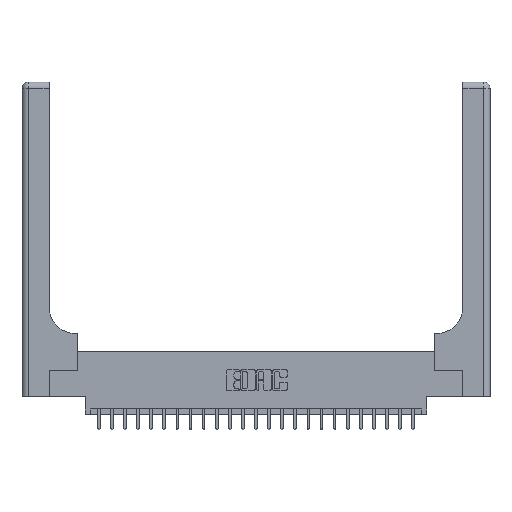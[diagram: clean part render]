
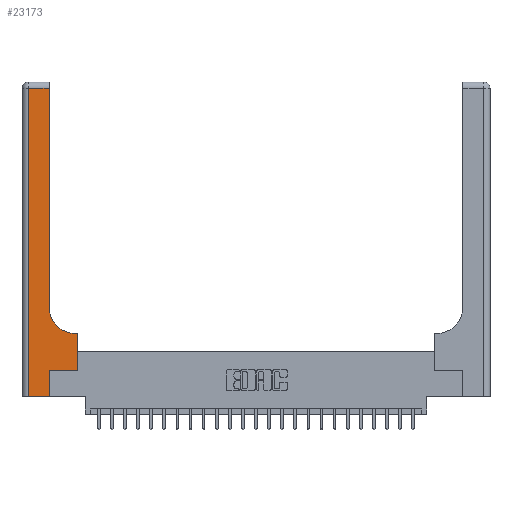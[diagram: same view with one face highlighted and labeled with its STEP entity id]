
A CAD part, top view. The second image highlights one B-rep face of the part: STEP entity #23173.
In plain terms, the highlighted planar face has unit normal (0, 0, 1).
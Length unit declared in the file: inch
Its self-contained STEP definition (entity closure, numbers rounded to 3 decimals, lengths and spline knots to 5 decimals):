
#363 = VECTOR ( 'NONE', #8334, 39.37008 ) ;
#521 = ORIENTED_EDGE ( 'NONE', *, *, #23786, .T. ) ;
#613 = CARTESIAN_POINT ( 'NONE',  ( 0.265, 0., 0.37 ) ) ;
#946 = VERTEX_POINT ( 'NONE', #2927 ) ;
#1017 = CARTESIAN_POINT ( 'NONE',  ( 0.26, 0.6, 0.37 ) ) ;
#1114 = AXIS2_PLACEMENT_3D ( 'NONE', #13629, #2464, #15475 ) ;
#1430 = EDGE_CURVE ( 'NONE', #2903, #22373, #16815, .T. ) ;
#2296 = CARTESIAN_POINT ( 'NONE',  ( 0.51, 0.6, 0.37 ) ) ;
#2464 = DIRECTION ( 'NONE',  ( 0., 0., -1. ) ) ;
#2522 = CARTESIAN_POINT ( 'NONE',  ( 0.26, 0.85, 0.37 ) ) ;
#2664 = ORIENTED_EDGE ( 'NONE', *, *, #9030, .T. ) ;
#2723 = LINE ( 'NONE', #8913, #23026 ) ;
#2903 = VERTEX_POINT ( 'NONE', #16398 ) ;
#2927 = CARTESIAN_POINT ( 'NONE',  ( 0.06, 0., 0.37 ) ) ;
#3464 = VECTOR ( 'NONE', #15496, 39.37008 ) ;
#3597 = CARTESIAN_POINT ( 'NONE',  ( 0.265, 0.25, 0.37 ) ) ;
#4015 = CARTESIAN_POINT ( 'NONE',  ( 0.06, 3., 0.37 ) ) ;
#4262 = CARTESIAN_POINT ( 'NONE',  ( 0.26, 3., 0.37 ) ) ;
#4944 = LINE ( 'NONE', #3597, #23441 ) ;
#5640 = FACE_OUTER_BOUND ( 'NONE', #9873, .T. ) ;
#5993 = EDGE_CURVE ( 'NONE', #946, #6659, #19519, .T. ) ;
#6459 = CARTESIAN_POINT ( 'NONE',  ( 0., 0., 0.37 ) ) ;
#6659 = VERTEX_POINT ( 'NONE', #19824 ) ;
#7111 = EDGE_CURVE ( 'NONE', #12697, #20676, #7682, .T. ) ;
#7594 = VECTOR ( 'NONE', #9465, 39.37008 ) ;
#7682 = LINE ( 'NONE', #4262, #8269 ) ;
#8269 = VECTOR ( 'NONE', #19010, 39.37008 ) ;
#8334 = DIRECTION ( 'NONE',  ( 1., 0., 0. ) ) ;
#8484 = CIRCLE ( 'NONE', #11244, 0.25 ) ;
#8913 = CARTESIAN_POINT ( 'NONE',  ( 0., 2.94, 0.37 ) ) ;
#9017 = LINE ( 'NONE', #613, #3464 ) ;
#9030 = EDGE_CURVE ( 'NONE', #18462, #14958, #4944, .T. ) ;
#9119 = ORIENTED_EDGE ( 'NONE', *, *, #5993, .T. ) ;
#9120 = EDGE_CURVE ( 'NONE', #14958, #2903, #22316, .T. ) ;
#9465 = DIRECTION ( 'NONE',  ( 0., 1., 0. ) ) ;
#9873 = EDGE_LOOP ( 'NONE', ( #22619, #17715, #521, #9119, #17446, #2664, #16441, #19282, #14045 ) ) ;
#10702 = CARTESIAN_POINT ( 'NONE',  ( 0.51, 0.85, 0.37 ) ) ;
#11056 = CARTESIAN_POINT ( 'NONE',  ( 0.265, 0.25, 0.37 ) ) ;
#11244 = AXIS2_PLACEMENT_3D ( 'NONE', #10702, #23586, #12565 ) ;
#11316 = CARTESIAN_POINT ( 'NONE',  ( 0.528, 0.25, 0.37 ) ) ;
#12344 = VERTEX_POINT ( 'NONE', #14685 ) ;
#12471 = DIRECTION ( 'NONE',  ( -1., 0., 0. ) ) ;
#12565 = DIRECTION ( 'NONE',  ( 1., 0., 0. ) ) ;
#12697 = VERTEX_POINT ( 'NONE', #2522 ) ;
#13629 = CARTESIAN_POINT ( 'NONE',  ( 0., 3., 0.37 ) ) ;
#14045 = ORIENTED_EDGE ( 'NONE', *, *, #19382, .T. ) ;
#14069 = DIRECTION ( 'NONE',  ( -1., 0., 0. ) ) ;
#14685 = CARTESIAN_POINT ( 'NONE',  ( 0.06, 2.94, 0.37 ) ) ;
#14958 = VERTEX_POINT ( 'NONE', #21641 ) ;
#15134 = DIRECTION ( 'NONE',  ( 0., -1., 0. ) ) ;
#15475 = DIRECTION ( 'NONE',  ( -1., 0., 0. ) ) ;
#15496 = DIRECTION ( 'NONE',  ( 0., 1., 0. ) ) ;
#16235 = EDGE_CURVE ( 'NONE', #20676, #12344, #2723, .T. ) ;
#16398 = CARTESIAN_POINT ( 'NONE',  ( 0.528, 0.6, 0.37 ) ) ;
#16441 = ORIENTED_EDGE ( 'NONE', *, *, #9120, .T. ) ;
#16815 = LINE ( 'NONE', #1017, #22313 ) ;
#17446 = ORIENTED_EDGE ( 'NONE', *, *, #19876, .T. ) ;
#17715 = ORIENTED_EDGE ( 'NONE', *, *, #16235, .T. ) ;
#18462 = VERTEX_POINT ( 'NONE', #11056 ) ;
#19010 = DIRECTION ( 'NONE',  ( 0., 1., 0. ) ) ;
#19282 = ORIENTED_EDGE ( 'NONE', *, *, #1430, .T. ) ;
#19382 = EDGE_CURVE ( 'NONE', #22373, #12697, #8484, .T. ) ;
#19519 = LINE ( 'NONE', #6459, #363 ) ;
#19824 = CARTESIAN_POINT ( 'NONE',  ( 0.265, 0., 0.37 ) ) ;
#19876 = EDGE_CURVE ( 'NONE', #6659, #18462, #9017, .T. ) ;
#20676 = VERTEX_POINT ( 'NONE', #23124 ) ;
#20963 = PLANE ( 'NONE',  #1114 ) ;
#21641 = CARTESIAN_POINT ( 'NONE',  ( 0.528, 0.25, 0.37 ) ) ;
#22313 = VECTOR ( 'NONE', #14069, 39.37008 ) ;
#22316 = LINE ( 'NONE', #11316, #7594 ) ;
#22373 = VERTEX_POINT ( 'NONE', #2296 ) ;
#22380 = VECTOR ( 'NONE', #15134, 39.37008 ) ;
#22619 = ORIENTED_EDGE ( 'NONE', *, *, #7111, .T. ) ;
#22951 = LINE ( 'NONE', #4015, #22380 ) ;
#23026 = VECTOR ( 'NONE', #12471, 39.37008 ) ;
#23124 = CARTESIAN_POINT ( 'NONE',  ( 0.26, 2.94, 0.37 ) ) ;
#23173 = ADVANCED_FACE ( 'NONE', ( #5640 ), #20963, .F. ) ;
#23441 = VECTOR ( 'NONE', #23950, 39.37008 ) ;
#23586 = DIRECTION ( 'NONE',  ( 0., 0., -1. ) ) ;
#23786 = EDGE_CURVE ( 'NONE', #12344, #946, #22951, .T. ) ;
#23950 = DIRECTION ( 'NONE',  ( 1., 0., 0. ) ) ;
